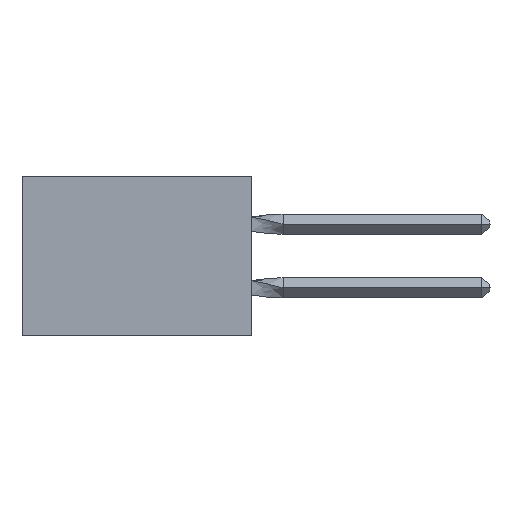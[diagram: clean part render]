
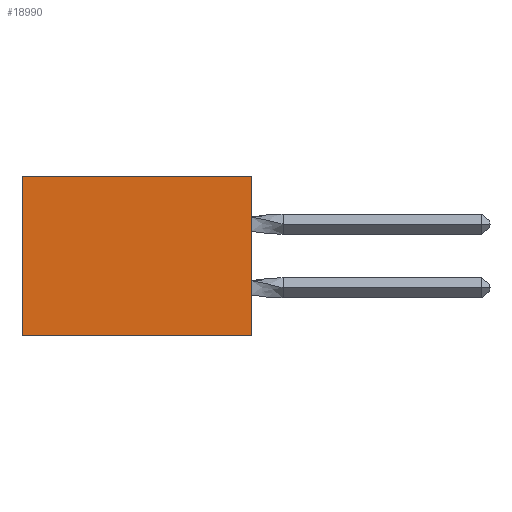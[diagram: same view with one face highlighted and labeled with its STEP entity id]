
A CAD part, left-side view. The second image highlights one B-rep face of the part: STEP entity #18990.
In plain terms, the highlighted planar face has unit normal (-1, 0, 0).
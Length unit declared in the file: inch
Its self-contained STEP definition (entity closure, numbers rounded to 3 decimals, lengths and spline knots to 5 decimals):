
#19 = LINE ( 'NONE', #14816, #11139 ) ;
#230 = ORIENTED_EDGE ( 'NONE', *, *, #9091, .F. ) ;
#1292 = EDGE_CURVE ( 'NONE', #13259, #21875, #19, .T. ) ;
#1536 = CARTESIAN_POINT ( 'NONE',  ( 0.305, 0., -0.5 ) ) ;
#2504 = CARTESIAN_POINT ( 'NONE',  ( 0.305, 0.72, -0.5 ) ) ;
#4651 = DIRECTION ( 'NONE',  ( 1., 0., 0. ) ) ;
#5166 = ORIENTED_EDGE ( 'NONE', *, *, #22468, .F. ) ;
#6440 = CARTESIAN_POINT ( 'NONE',  ( 0.305, 0.72, -0.5 ) ) ;
#7749 = ORIENTED_EDGE ( 'NONE', *, *, #1292, .T. ) ;
#8313 = DIRECTION ( 'NONE',  ( 0., 0., -1. ) ) ;
#8759 = VECTOR ( 'NONE', #20698, 39.37008 ) ;
#9091 = EDGE_CURVE ( 'NONE', #13259, #14395, #22055, .T. ) ;
#10260 = PLANE ( 'NONE',  #14598 ) ;
#10799 = CARTESIAN_POINT ( 'NONE',  ( 0.305, 0., -0.5 ) ) ;
#11139 = VECTOR ( 'NONE', #22716, 39.37008 ) ;
#11647 = CARTESIAN_POINT ( 'NONE',  ( 0.305, 0.72, 0. ) ) ;
#12277 = CARTESIAN_POINT ( 'NONE',  ( 0.305, 0., -0.5 ) ) ;
#13031 = CARTESIAN_POINT ( 'NONE',  ( 0.305, 0., -0.5 ) ) ;
#13259 = VERTEX_POINT ( 'NONE', #15771 ) ;
#14395 = VERTEX_POINT ( 'NONE', #13031 ) ;
#14556 = FACE_OUTER_BOUND ( 'NONE', #19814, .T. ) ;
#14598 = AXIS2_PLACEMENT_3D ( 'NONE', #12277, #4651, #15884 ) ;
#14670 = LINE ( 'NONE', #10799, #17695 ) ;
#14816 = CARTESIAN_POINT ( 'NONE',  ( 0.305, 0., 0. ) ) ;
#15771 = CARTESIAN_POINT ( 'NONE',  ( 0.305, 0., 0. ) ) ;
#15884 = DIRECTION ( 'NONE',  ( 0., 0., -1. ) ) ;
#17448 = ORIENTED_EDGE ( 'NONE', *, *, #20846, .T. ) ;
#17695 = VECTOR ( 'NONE', #22418, 39.37008 ) ;
#18990 = ADVANCED_FACE ( 'NONE', ( #14556 ), #10260, .F. ) ;
#19814 = EDGE_LOOP ( 'NONE', ( #17448, #5166, #230, #7749 ) ) ;
#20548 = LINE ( 'NONE', #2504, #21439 ) ;
#20698 = DIRECTION ( 'NONE',  ( 0., 0., -1. ) ) ;
#20846 = EDGE_CURVE ( 'NONE', #21875, #21984, #20548, .T. ) ;
#21439 = VECTOR ( 'NONE', #8313, 39.37008 ) ;
#21875 = VERTEX_POINT ( 'NONE', #11647 ) ;
#21984 = VERTEX_POINT ( 'NONE', #6440 ) ;
#22055 = LINE ( 'NONE', #1536, #8759 ) ;
#22418 = DIRECTION ( 'NONE',  ( 0., 1., 0. ) ) ;
#22468 = EDGE_CURVE ( 'NONE', #14395, #21984, #14670, .T. ) ;
#22716 = DIRECTION ( 'NONE',  ( 0., 1., 0. ) ) ;
